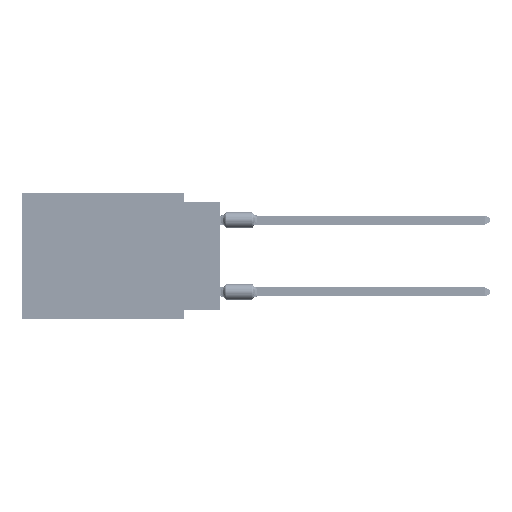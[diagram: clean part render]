
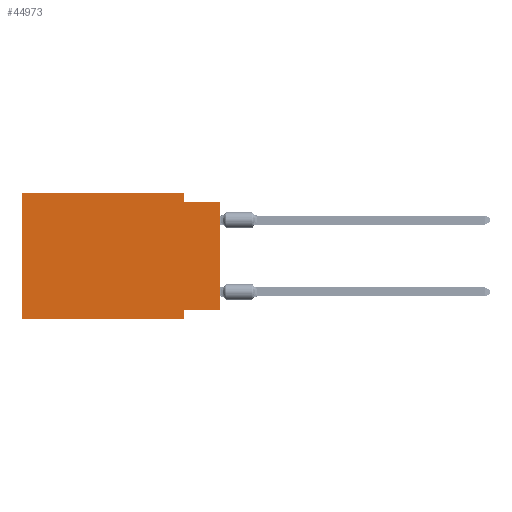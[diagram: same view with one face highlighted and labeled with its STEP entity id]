
A CAD part, left-side view. The second image highlights one B-rep face of the part: STEP entity #44973.
In plain terms, the highlighted planar face has unit normal (-1, 0, 0).
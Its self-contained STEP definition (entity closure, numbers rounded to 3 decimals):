
#1803 = EDGE_CURVE ( 'NONE', #23755, #49233, #27870, .T. ) ;
#3966 = CARTESIAN_POINT ( 'NONE',  ( 0., 0., -0.635 ) ) ;
#4945 = ORIENTED_EDGE ( 'NONE', *, *, #1803, .F. ) ;
#5607 = CARTESIAN_POINT ( 'NONE',  ( 0., 13.97, 0. ) ) ;
#6467 = LINE ( 'NONE', #44847, #27443 ) ;
#6850 = DIRECTION ( 'NONE',  ( 0., -1., 0. ) ) ;
#7215 = LINE ( 'NONE', #51082, #11224 ) ;
#7314 = PLANE ( 'NONE',  #43456 ) ;
#9266 = CARTESIAN_POINT ( 'NONE',  ( 0., 13.97, -8.89 ) ) ;
#10664 = ORIENTED_EDGE ( 'NONE', *, *, #55998, .F. ) ;
#11224 = VECTOR ( 'NONE', #6850, 1000. ) ;
#13144 = DIRECTION ( 'NONE',  ( 1., 0., 0. ) ) ;
#15139 = EDGE_CURVE ( 'NONE', #17298, #46074, #22542, .T. ) ;
#17067 = DIRECTION ( 'NONE',  ( 0., 1., 0. ) ) ;
#17298 = VERTEX_POINT ( 'NONE', #36262 ) ;
#17947 = EDGE_CURVE ( 'NONE', #68016, #67300, #6467, .T. ) ;
#18790 = CARTESIAN_POINT ( 'NONE',  ( 0., 2.54, -8.255 ) ) ;
#19253 = EDGE_CURVE ( 'NONE', #49233, #68016, #7215, .T. ) ;
#20381 = ORIENTED_EDGE ( 'NONE', *, *, #19253, .F. ) ;
#21160 = VECTOR ( 'NONE', #17067, 1000. ) ;
#21467 = VERTEX_POINT ( 'NONE', #55932 ) ;
#21683 = CARTESIAN_POINT ( 'NONE',  ( 0., 0., 0. ) ) ;
#22542 = LINE ( 'NONE', #67143, #21160 ) ;
#23755 = VERTEX_POINT ( 'NONE', #37336 ) ;
#24975 = EDGE_LOOP ( 'NONE', ( #37556, #28168, #68087, #20381, #4945, #67209, #10664, #46754 ) ) ;
#26597 = VECTOR ( 'NONE', #31193, 1000. ) ;
#26793 = CARTESIAN_POINT ( 'NONE',  ( 0., 2.54, 0. ) ) ;
#27443 = VECTOR ( 'NONE', #39390, 1000. ) ;
#27870 = LINE ( 'NONE', #5607, #30183 ) ;
#28168 = ORIENTED_EDGE ( 'NONE', *, *, #44135, .F. ) ;
#30183 = VECTOR ( 'NONE', #49834, 1000. ) ;
#31193 = DIRECTION ( 'NONE',  ( 0., -1., 0. ) ) ;
#31645 = EDGE_CURVE ( 'NONE', #23755, #21467, #35953, .T. ) ;
#33168 = VECTOR ( 'NONE', #44004, 1000. ) ;
#35405 = CARTESIAN_POINT ( 'NONE',  ( 0., 2.54, -8.89 ) ) ;
#35953 = LINE ( 'NONE', #9266, #26597 ) ;
#36262 = CARTESIAN_POINT ( 'NONE',  ( 0., 0., -8.255 ) ) ;
#37336 = CARTESIAN_POINT ( 'NONE',  ( 0., 13.97, -8.89 ) ) ;
#37556 = ORIENTED_EDGE ( 'NONE', *, *, #47654, .T. ) ;
#39390 = DIRECTION ( 'NONE',  ( 0., 0., -1. ) ) ;
#40030 = VECTOR ( 'NONE', #58793, 1000. ) ;
#40477 = DIRECTION ( 'NONE',  ( 0., -1., 0. ) ) ;
#43456 = AXIS2_PLACEMENT_3D ( 'NONE', #69412, #13144, #46034 ) ;
#43862 = CARTESIAN_POINT ( 'NONE',  ( 0., 2.54, -0.635 ) ) ;
#44004 = DIRECTION ( 'NONE',  ( 0., 0., 1. ) ) ;
#44135 = EDGE_CURVE ( 'NONE', #67300, #56124, #57282, .T. ) ;
#44847 = CARTESIAN_POINT ( 'NONE',  ( 0., 2.54, 0. ) ) ;
#44973 = ADVANCED_FACE ( 'NONE', ( #57374 ), #7314, .F. ) ;
#46034 = DIRECTION ( 'NONE',  ( 0., 0., -1. ) ) ;
#46074 = VERTEX_POINT ( 'NONE', #18790 ) ;
#46732 = LINE ( 'NONE', #35405, #40030 ) ;
#46754 = ORIENTED_EDGE ( 'NONE', *, *, #15139, .F. ) ;
#47654 = EDGE_CURVE ( 'NONE', #17298, #56124, #71748, .T. ) ;
#49233 = VERTEX_POINT ( 'NONE', #51554 ) ;
#49416 = VECTOR ( 'NONE', #40477, 1000. ) ;
#49834 = DIRECTION ( 'NONE',  ( 0., 0., 1. ) ) ;
#51082 = CARTESIAN_POINT ( 'NONE',  ( 0., 13.97, 0. ) ) ;
#51437 = CARTESIAN_POINT ( 'NONE',  ( 0., 0., -0.635 ) ) ;
#51554 = CARTESIAN_POINT ( 'NONE',  ( 0., 13.97, 0. ) ) ;
#55932 = CARTESIAN_POINT ( 'NONE',  ( 0., 2.54, -8.89 ) ) ;
#55998 = EDGE_CURVE ( 'NONE', #46074, #21467, #46732, .T. ) ;
#56124 = VERTEX_POINT ( 'NONE', #3966 ) ;
#57282 = LINE ( 'NONE', #51437, #49416 ) ;
#57374 = FACE_OUTER_BOUND ( 'NONE', #24975, .T. ) ;
#58793 = DIRECTION ( 'NONE',  ( 0., 0., -1. ) ) ;
#67143 = CARTESIAN_POINT ( 'NONE',  ( 0., 0., -8.255 ) ) ;
#67209 = ORIENTED_EDGE ( 'NONE', *, *, #31645, .T. ) ;
#67300 = VERTEX_POINT ( 'NONE', #43862 ) ;
#68016 = VERTEX_POINT ( 'NONE', #26793 ) ;
#68087 = ORIENTED_EDGE ( 'NONE', *, *, #17947, .F. ) ;
#69412 = CARTESIAN_POINT ( 'NONE',  ( 0., 13.97, 0. ) ) ;
#71748 = LINE ( 'NONE', #21683, #33168 ) ;
